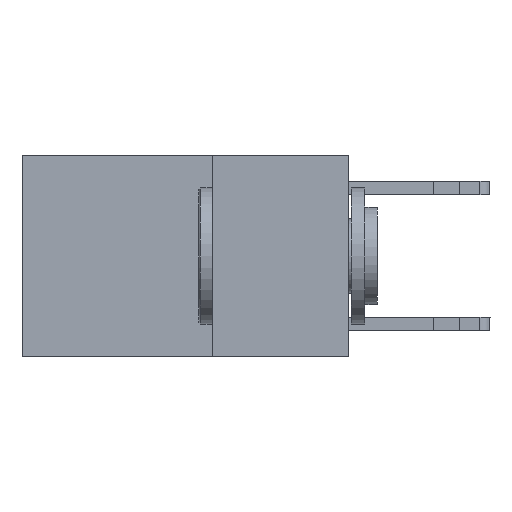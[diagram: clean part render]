
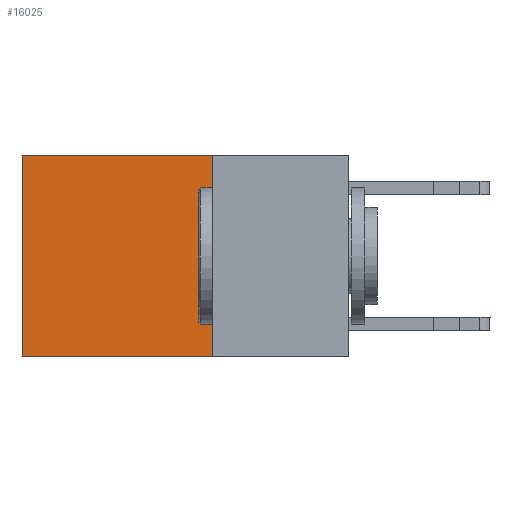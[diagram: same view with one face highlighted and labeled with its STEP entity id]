
A CAD part, left-side view. The second image highlights one B-rep face of the part: STEP entity #16025.
In plain terms, the highlighted planar face has unit normal (-1, 0, 0).
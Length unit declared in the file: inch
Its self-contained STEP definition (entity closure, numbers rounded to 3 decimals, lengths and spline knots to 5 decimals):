
#3 = EDGE_CURVE ( 'NONE', #21357, #13419, #12486, .T. ) ;
#145 = VECTOR ( 'NONE', #16468, 39.37008 ) ;
#457 = LINE ( 'NONE', #18648, #145 ) ;
#521 = EDGE_CURVE ( 'NONE', #21357, #12389, #9230, .T. ) ;
#1977 = ORIENTED_EDGE ( 'NONE', *, *, #521, .F. ) ;
#3096 = CARTESIAN_POINT ( 'NONE',  ( 0.2625, 0.25, 0. ) ) ;
#4162 = CARTESIAN_POINT ( 'NONE',  ( 0.2625, 0.6, 0. ) ) ;
#5308 = EDGE_CURVE ( 'NONE', #12389, #16247, #457, .T. ) ;
#5790 = DIRECTION ( 'NONE',  ( 0., 0., -1. ) ) ;
#7886 = EDGE_LOOP ( 'NONE', ( #9581, #12493, #1977, #14978 ) ) ;
#8834 = CARTESIAN_POINT ( 'NONE',  ( 0.2625, 0.6, -0.37 ) ) ;
#9227 = VECTOR ( 'NONE', #5790, 39.37008 ) ;
#9230 = LINE ( 'NONE', #17873, #9227 ) ;
#9581 = ORIENTED_EDGE ( 'NONE', *, *, #22626, .T. ) ;
#10946 = CARTESIAN_POINT ( 'NONE',  ( 0.2625, 0.25, 0. ) ) ;
#11990 = AXIS2_PLACEMENT_3D ( 'NONE', #13062, #12990, #12934 ) ;
#12389 = VERTEX_POINT ( 'NONE', #21368 ) ;
#12458 = VECTOR ( 'NONE', #21197, 39.37008 ) ;
#12486 = LINE ( 'NONE', #3096, #12458 ) ;
#12493 = ORIENTED_EDGE ( 'NONE', *, *, #5308, .F. ) ;
#12934 = DIRECTION ( 'NONE',  ( 0., 0., -1. ) ) ;
#12990 = DIRECTION ( 'NONE',  ( 1., 0., 0. ) ) ;
#13062 = CARTESIAN_POINT ( 'NONE',  ( 0.2625, 0.25, 0. ) ) ;
#13192 = PLANE ( 'NONE',  #11990 ) ;
#13419 = VERTEX_POINT ( 'NONE', #4162 ) ;
#14978 = ORIENTED_EDGE ( 'NONE', *, *, #3, .T. ) ;
#16025 = ADVANCED_FACE ( 'NONE', ( #21021 ), #13192, .F. ) ;
#16247 = VERTEX_POINT ( 'NONE', #8834 ) ;
#16419 = LINE ( 'NONE', #22869, #16446 ) ;
#16446 = VECTOR ( 'NONE', #23018, 39.37008 ) ;
#16468 = DIRECTION ( 'NONE',  ( 0., 1., 0. ) ) ;
#17873 = CARTESIAN_POINT ( 'NONE',  ( 0.2625, 0.25, 0. ) ) ;
#18648 = CARTESIAN_POINT ( 'NONE',  ( 0.2625, 0.25, -0.37 ) ) ;
#21021 = FACE_OUTER_BOUND ( 'NONE', #7886, .T. ) ;
#21197 = DIRECTION ( 'NONE',  ( 0., 1., 0. ) ) ;
#21357 = VERTEX_POINT ( 'NONE', #10946 ) ;
#21368 = CARTESIAN_POINT ( 'NONE',  ( 0.2625, 0.25, -0.37 ) ) ;
#22626 = EDGE_CURVE ( 'NONE', #13419, #16247, #16419, .T. ) ;
#22869 = CARTESIAN_POINT ( 'NONE',  ( 0.2625, 0.6, 0. ) ) ;
#23018 = DIRECTION ( 'NONE',  ( 0., 0., -1. ) ) ;
